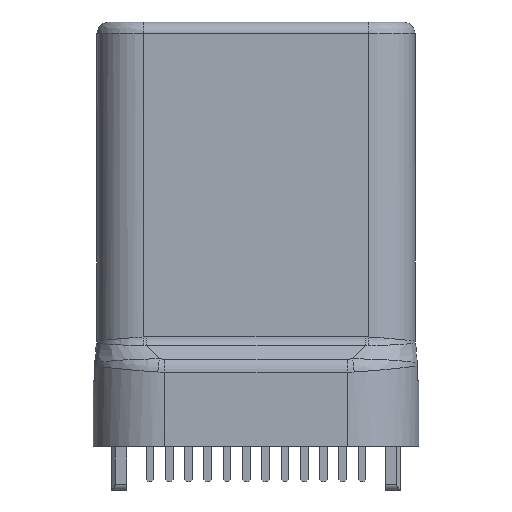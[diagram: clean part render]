
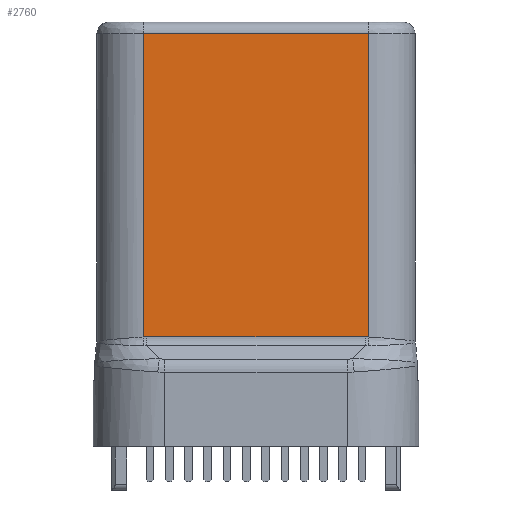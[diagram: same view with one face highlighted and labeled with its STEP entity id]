
A CAD part, front view. The second image highlights one B-rep face of the part: STEP entity #2760.
In plain terms, the highlighted planar face has unit normal (0, -1, 0).
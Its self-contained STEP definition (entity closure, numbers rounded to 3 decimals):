
#1074 = DIRECTION ( 'NONE',  ( 0., -1., 0. ) ) ;
#2136 = EDGE_LOOP ( 'NONE', ( #22855, #51056, #39142, #35804, #12627, #11297 ) ) ;
#2760 = ADVANCED_FACE ( 'NONE', ( #5827 ), #62686, .T. ) ;
#2815 = EDGE_CURVE ( 'NONE', #47114, #42054, #41191, .T. ) ;
#5827 = FACE_OUTER_BOUND ( 'NONE', #2136, .T. ) ;
#6542 = CARTESIAN_POINT ( 'NONE',  ( 0., -1.2, -4.05 ) ) ;
#7893 = CARTESIAN_POINT ( 'NONE',  ( 0., -1.2, -0.2 ) ) ;
#9930 = VERTEX_POINT ( 'NONE', #50305 ) ;
#10712 = DIRECTION ( 'NONE',  ( 0., 0., -1. ) ) ;
#10824 = EDGE_CURVE ( 'NONE', #23242, #14849, #25289, .T. ) ;
#11062 = CARTESIAN_POINT ( 'NONE',  ( -2.925, -1.2, -4.05 ) ) ;
#11297 = ORIENTED_EDGE ( 'NONE', *, *, #10824, .T. ) ;
#12627 = ORIENTED_EDGE ( 'NONE', *, *, #46235, .T. ) ;
#13314 = CARTESIAN_POINT ( 'NONE',  ( 2.925, -1.2, -4.05 ) ) ;
#14849 = VERTEX_POINT ( 'NONE', #45784 ) ;
#15968 = CARTESIAN_POINT ( 'NONE',  ( 2.838, -1.2, -8.063 ) ) ;
#16048 = CARTESIAN_POINT ( 'NONE',  ( -2.925, -1.2, -0.2 ) ) ;
#16224 = VECTOR ( 'NONE', #23285, 1000. ) ;
#17697 = VERTEX_POINT ( 'NONE', #16048 ) ;
#19127 = DIRECTION ( 'NONE',  ( 0., 0., 1. ) ) ;
#19544 = LINE ( 'NONE', #7893, #31982 ) ;
#22855 = ORIENTED_EDGE ( 'NONE', *, *, #28478, .T. ) ;
#23242 = VERTEX_POINT ( 'NONE', #31738 ) ;
#23285 = DIRECTION ( 'NONE',  ( 1., 0., -0.025 ) ) ;
#24688 = DIRECTION ( 'NONE',  ( -1., 0., 0. ) ) ;
#25289 = LINE ( 'NONE', #13314, #71005 ) ;
#26130 = DIRECTION ( 'NONE',  ( 1., 0., 0.025 ) ) ;
#28478 = EDGE_CURVE ( 'NONE', #14849, #17697, #19544, .T. ) ;
#30564 = LINE ( 'NONE', #52803, #16224 ) ;
#31227 = CARTESIAN_POINT ( 'NONE',  ( -2.925, -1.2, -8.065 ) ) ;
#31738 = CARTESIAN_POINT ( 'NONE',  ( 2.925, -1.2, -8.065 ) ) ;
#31945 = LINE ( 'NONE', #31227, #58318 ) ;
#31982 = VECTOR ( 'NONE', #24688, 1000. ) ;
#33095 = EDGE_CURVE ( 'NONE', #17697, #9930, #66469, .T. ) ;
#34998 = DIRECTION ( 'NONE',  ( 0., 0., -1. ) ) ;
#35804 = ORIENTED_EDGE ( 'NONE', *, *, #2815, .T. ) ;
#39142 = ORIENTED_EDGE ( 'NONE', *, *, #43338, .T. ) ;
#40785 = CARTESIAN_POINT ( 'NONE',  ( -2.838, -1.2, -8.063 ) ) ;
#41191 = LINE ( 'NONE', #52852, #60773 ) ;
#42054 = VERTEX_POINT ( 'NONE', #15968 ) ;
#43338 = EDGE_CURVE ( 'NONE', #9930, #47114, #31945, .T. ) ;
#44517 = AXIS2_PLACEMENT_3D ( 'NONE', #6542, #1074, #34998 ) ;
#45784 = CARTESIAN_POINT ( 'NONE',  ( 2.925, -1.2, -0.2 ) ) ;
#46235 = EDGE_CURVE ( 'NONE', #42054, #23242, #30564, .T. ) ;
#46331 = VECTOR ( 'NONE', #10712, 1000. ) ;
#47114 = VERTEX_POINT ( 'NONE', #40785 ) ;
#47733 = DIRECTION ( 'NONE',  ( 1., 0., 0. ) ) ;
#50305 = CARTESIAN_POINT ( 'NONE',  ( -2.925, -1.2, -8.065 ) ) ;
#51056 = ORIENTED_EDGE ( 'NONE', *, *, #33095, .T. ) ;
#52803 = CARTESIAN_POINT ( 'NONE',  ( 2.838, -1.2, -8.063 ) ) ;
#52852 = CARTESIAN_POINT ( 'NONE',  ( 0., -1.2, -8.063 ) ) ;
#58318 = VECTOR ( 'NONE', #26130, 1000. ) ;
#60773 = VECTOR ( 'NONE', #47733, 1000. ) ;
#62686 = PLANE ( 'NONE',  #44517 ) ;
#66469 = LINE ( 'NONE', #11062, #46331 ) ;
#71005 = VECTOR ( 'NONE', #19127, 1000. ) ;
